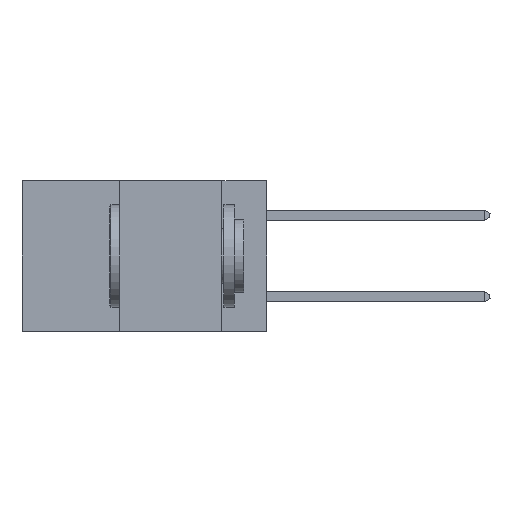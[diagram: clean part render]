
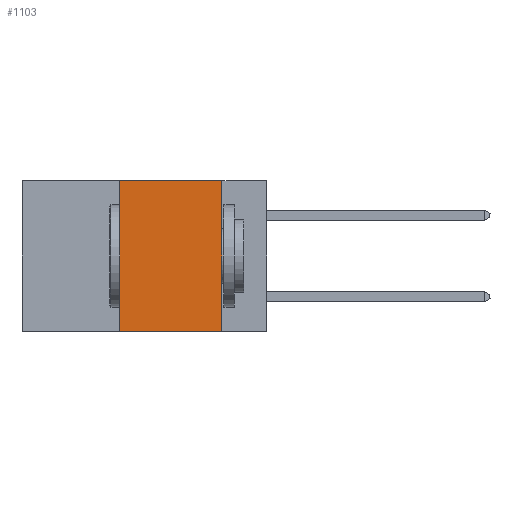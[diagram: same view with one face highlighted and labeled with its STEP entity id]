
A CAD part, left-side view. The second image highlights one B-rep face of the part: STEP entity #1103.
In plain terms, the highlighted planar face has unit normal (-1, 0, 0).
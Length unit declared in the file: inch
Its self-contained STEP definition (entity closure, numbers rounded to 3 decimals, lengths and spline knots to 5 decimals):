
#1103 = ADVANCED_FACE ( 'NONE', ( #19914 ), #2966, .F. ) ;
#2966 = PLANE ( 'NONE',  #46041 ) ;
#3336 = DIRECTION ( 'NONE',  ( 0., 0., 1. ) ) ;
#3962 = ORIENTED_EDGE ( 'NONE', *, *, #9180, .F. ) ;
#4082 = VECTOR ( 'NONE', #31790, 39.37008 ) ;
#6531 = DIRECTION ( 'NONE',  ( 0., -1., 0. ) ) ;
#9180 = EDGE_CURVE ( 'NONE', #23606, #14219, #21297, .T. ) ;
#9186 = LINE ( 'NONE', #31942, #4082 ) ;
#14107 = CARTESIAN_POINT ( 'NONE',  ( 0., 0.11, -0.37 ) ) ;
#14219 = VERTEX_POINT ( 'NONE', #23227 ) ;
#18095 = CARTESIAN_POINT ( 'NONE',  ( 0., 0.36, -0.37 ) ) ;
#19914 = FACE_OUTER_BOUND ( 'NONE', #24631, .T. ) ;
#20138 = LINE ( 'NONE', #29191, #25761 ) ;
#20452 = ORIENTED_EDGE ( 'NONE', *, *, #21120, .F. ) ;
#21120 = EDGE_CURVE ( 'NONE', #14219, #27841, #9186, .T. ) ;
#21297 = LINE ( 'NONE', #42088, #43386 ) ;
#21658 = VECTOR ( 'NONE', #6531, 39.37008 ) ;
#23227 = CARTESIAN_POINT ( 'NONE',  ( 0., 0.11, 0. ) ) ;
#23606 = VERTEX_POINT ( 'NONE', #39762 ) ;
#24631 = EDGE_LOOP ( 'NONE', ( #20452, #3962, #32884, #33128 ) ) ;
#25761 = VECTOR ( 'NONE', #3336, 39.37008 ) ;
#27841 = VERTEX_POINT ( 'NONE', #14107 ) ;
#28149 = CARTESIAN_POINT ( 'NONE',  ( 0., 0.6, -0.37 ) ) ;
#28211 = DIRECTION ( 'NONE',  ( 0., 0., -1. ) ) ;
#29191 = CARTESIAN_POINT ( 'NONE',  ( 0., 0.36, 0. ) ) ;
#31054 = DIRECTION ( 'NONE',  ( 1., 0., 0. ) ) ;
#31790 = DIRECTION ( 'NONE',  ( 0., 0., -1. ) ) ;
#31942 = CARTESIAN_POINT ( 'NONE',  ( 0., 0.11, 0. ) ) ;
#32884 = ORIENTED_EDGE ( 'NONE', *, *, #38435, .F. ) ;
#33128 = ORIENTED_EDGE ( 'NONE', *, *, #35350, .T. ) ;
#35350 = EDGE_CURVE ( 'NONE', #46258, #27841, #44836, .T. ) ;
#38435 = EDGE_CURVE ( 'NONE', #46258, #23606, #20138, .T. ) ;
#39762 = CARTESIAN_POINT ( 'NONE',  ( 0., 0.36, 0. ) ) ;
#42088 = CARTESIAN_POINT ( 'NONE',  ( 0., 0.6, 0. ) ) ;
#42378 = DIRECTION ( 'NONE',  ( 0., -1., 0. ) ) ;
#43386 = VECTOR ( 'NONE', #42378, 39.37008 ) ;
#44836 = LINE ( 'NONE', #28149, #21658 ) ;
#45622 = CARTESIAN_POINT ( 'NONE',  ( 0., 0.6, 0. ) ) ;
#46041 = AXIS2_PLACEMENT_3D ( 'NONE', #45622, #31054, #28211 ) ;
#46258 = VERTEX_POINT ( 'NONE', #18095 ) ;
